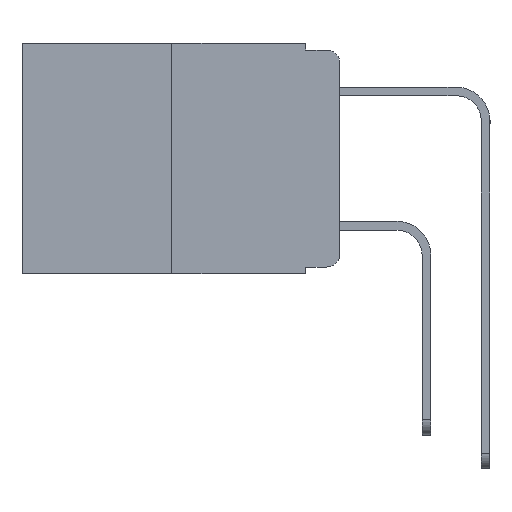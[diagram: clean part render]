
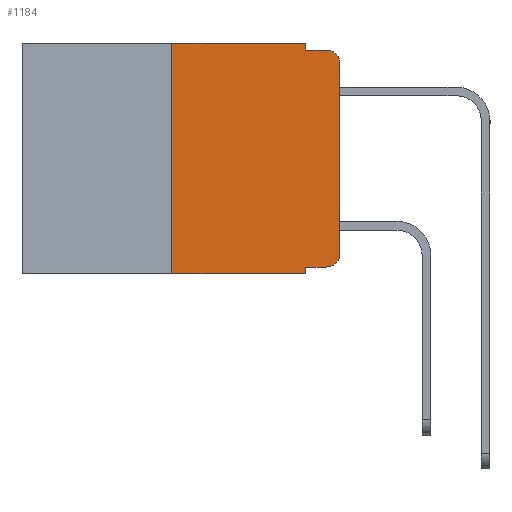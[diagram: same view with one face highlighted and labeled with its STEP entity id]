
A CAD part, left-side view. The second image highlights one B-rep face of the part: STEP entity #1184.
In plain terms, the highlighted planar face has unit normal (-1, 0, 0).
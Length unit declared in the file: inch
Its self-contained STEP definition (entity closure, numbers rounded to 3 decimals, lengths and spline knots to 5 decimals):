
#219 = VERTEX_POINT ( 'NONE', #6399 ) ;
#426 = DIRECTION ( 'NONE',  ( 0., 0., 1. ) ) ;
#668 = EDGE_LOOP ( 'NONE', ( #4112, #11697, #12243, #10073, #11960, #9664, #2166, #1937, #10912, #15473 ) ) ;
#960 = VECTOR ( 'NONE', #4461, 39.37008 ) ;
#1008 = CARTESIAN_POINT ( 'NONE',  ( 0., 0.051, -0.01 ) ) ;
#1034 = EDGE_CURVE ( 'NONE', #2214, #12035, #7210, .T. ) ;
#1060 = FACE_OUTER_BOUND ( 'NONE', #668, .T. ) ;
#1184 = ADVANCED_FACE ( 'NONE', ( #1060 ), #11870, .F. ) ;
#1248 = VERTEX_POINT ( 'NONE', #2915 ) ;
#1490 = LINE ( 'NONE', #2343, #12037 ) ;
#1596 = VERTEX_POINT ( 'NONE', #1008 ) ;
#1782 = VERTEX_POINT ( 'NONE', #12039 ) ;
#1937 = ORIENTED_EDGE ( 'NONE', *, *, #6773, .F. ) ;
#1975 = CARTESIAN_POINT ( 'NONE',  ( 0., 0.02, -0.03 ) ) ;
#2166 = ORIENTED_EDGE ( 'NONE', *, *, #7010, .T. ) ;
#2214 = VERTEX_POINT ( 'NONE', #8139 ) ;
#2343 = CARTESIAN_POINT ( 'NONE',  ( 0., 0.051, 0. ) ) ;
#2454 = VECTOR ( 'NONE', #12925, 39.37008 ) ;
#2482 = CARTESIAN_POINT ( 'NONE',  ( 0., 0.051, -0.333 ) ) ;
#2485 = DIRECTION ( 'NONE',  ( 0., -1., 0. ) ) ;
#2839 = VERTEX_POINT ( 'NONE', #2482 ) ;
#2915 = CARTESIAN_POINT ( 'NONE',  ( 0., 0.02, -0.333 ) ) ;
#2952 = EDGE_CURVE ( 'NONE', #1248, #4458, #9739, .T. ) ;
#3484 = DIRECTION ( 'NONE',  ( 0., 0., -1. ) ) ;
#3716 = DIRECTION ( 'NONE',  ( 1., 0., 0. ) ) ;
#3717 = CARTESIAN_POINT ( 'NONE',  ( 0., 0.473, 0. ) ) ;
#4112 = ORIENTED_EDGE ( 'NONE', *, *, #12880, .T. ) ;
#4139 = DIRECTION ( 'NONE',  ( 0., 0., -1. ) ) ;
#4273 = DIRECTION ( 'NONE',  ( -1., 0., 0. ) ) ;
#4321 = CARTESIAN_POINT ( 'NONE',  ( 0., 0.02, -0.313 ) ) ;
#4362 = VERTEX_POINT ( 'NONE', #9790 ) ;
#4458 = VERTEX_POINT ( 'NONE', #6337 ) ;
#4461 = DIRECTION ( 'NONE',  ( 0., -1., 0. ) ) ;
#5342 = DIRECTION ( 'NONE',  ( 0., 0., 1. ) ) ;
#5611 = VECTOR ( 'NONE', #5342, 39.37008 ) ;
#5639 = VECTOR ( 'NONE', #5933, 39.37008 ) ;
#5848 = EDGE_CURVE ( 'NONE', #2839, #1248, #10043, .T. ) ;
#5933 = DIRECTION ( 'NONE',  ( 0., 0., -1. ) ) ;
#6082 = LINE ( 'NONE', #8596, #5639 ) ;
#6337 = CARTESIAN_POINT ( 'NONE',  ( 0., 0., -0.313 ) ) ;
#6399 = CARTESIAN_POINT ( 'NONE',  ( 0., 0.25, -0.343 ) ) ;
#6604 = DIRECTION ( 'NONE',  ( 0., 0., -1. ) ) ;
#6773 = EDGE_CURVE ( 'NONE', #2839, #1782, #6082, .T. ) ;
#6877 = CARTESIAN_POINT ( 'NONE',  ( 0., 0.051, 0. ) ) ;
#7010 = EDGE_CURVE ( 'NONE', #219, #1782, #9803, .T. ) ;
#7210 = LINE ( 'NONE', #9459, #10248 ) ;
#7686 = EDGE_CURVE ( 'NONE', #219, #2214, #9181, .T. ) ;
#8139 = CARTESIAN_POINT ( 'NONE',  ( 0., 0.25, 0. ) ) ;
#8276 = VERTEX_POINT ( 'NONE', #16850 ) ;
#8596 = CARTESIAN_POINT ( 'NONE',  ( 0., 0.051, 0. ) ) ;
#9181 = LINE ( 'NONE', #11950, #5611 ) ;
#9417 = EDGE_CURVE ( 'NONE', #12035, #1596, #1490, .T. ) ;
#9459 = CARTESIAN_POINT ( 'NONE',  ( 0., 0.473, 0. ) ) ;
#9664 = ORIENTED_EDGE ( 'NONE', *, *, #7686, .F. ) ;
#9739 = CIRCLE ( 'NONE', #12643, 0.02 ) ;
#9790 = CARTESIAN_POINT ( 'NONE',  ( 0., 0.02, -0.01 ) ) ;
#9803 = LINE ( 'NONE', #16621, #2454 ) ;
#10043 = LINE ( 'NONE', #10705, #13078 ) ;
#10073 = ORIENTED_EDGE ( 'NONE', *, *, #9417, .F. ) ;
#10248 = VECTOR ( 'NONE', #11378, 39.37008 ) ;
#10258 = CARTESIAN_POINT ( 'NONE',  ( 0., 0., 0. ) ) ;
#10268 = EDGE_CURVE ( 'NONE', #1596, #4362, #12009, .T. ) ;
#10563 = AXIS2_PLACEMENT_3D ( 'NONE', #1975, #11590, #3484 ) ;
#10705 = CARTESIAN_POINT ( 'NONE',  ( 0., 0.051, -0.333 ) ) ;
#10912 = ORIENTED_EDGE ( 'NONE', *, *, #5848, .T. ) ;
#11062 = CARTESIAN_POINT ( 'NONE',  ( 0., 0.051, -0.01 ) ) ;
#11163 = EDGE_CURVE ( 'NONE', #8276, #4362, #16070, .T. ) ;
#11378 = DIRECTION ( 'NONE',  ( 0., -1., 0. ) ) ;
#11590 = DIRECTION ( 'NONE',  ( -1., 0., 0. ) ) ;
#11697 = ORIENTED_EDGE ( 'NONE', *, *, #11163, .T. ) ;
#11870 = PLANE ( 'NONE',  #13376 ) ;
#11950 = CARTESIAN_POINT ( 'NONE',  ( 0., 0.25, 0. ) ) ;
#11960 = ORIENTED_EDGE ( 'NONE', *, *, #1034, .F. ) ;
#12009 = LINE ( 'NONE', #11062, #960 ) ;
#12035 = VERTEX_POINT ( 'NONE', #6877 ) ;
#12037 = VECTOR ( 'NONE', #14358, 39.37008 ) ;
#12039 = CARTESIAN_POINT ( 'NONE',  ( 0., 0.051, -0.343 ) ) ;
#12141 = VECTOR ( 'NONE', #426, 39.37008 ) ;
#12243 = ORIENTED_EDGE ( 'NONE', *, *, #10268, .F. ) ;
#12643 = AXIS2_PLACEMENT_3D ( 'NONE', #4321, #4273, #4139 ) ;
#12880 = EDGE_CURVE ( 'NONE', #4458, #8276, #15460, .T. ) ;
#12925 = DIRECTION ( 'NONE',  ( 0., -1., 0. ) ) ;
#13078 = VECTOR ( 'NONE', #2485, 39.37008 ) ;
#13376 = AXIS2_PLACEMENT_3D ( 'NONE', #3717, #3716, #6604 ) ;
#14358 = DIRECTION ( 'NONE',  ( 0., 0., -1. ) ) ;
#15460 = LINE ( 'NONE', #10258, #12141 ) ;
#15473 = ORIENTED_EDGE ( 'NONE', *, *, #2952, .T. ) ;
#16070 = CIRCLE ( 'NONE', #10563, 0.02 ) ;
#16621 = CARTESIAN_POINT ( 'NONE',  ( 0., 0.473, -0.343 ) ) ;
#16850 = CARTESIAN_POINT ( 'NONE',  ( 0., 0., -0.03 ) ) ;
